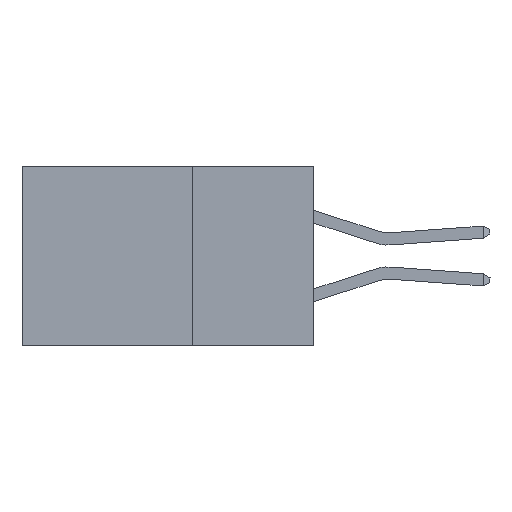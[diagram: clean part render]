
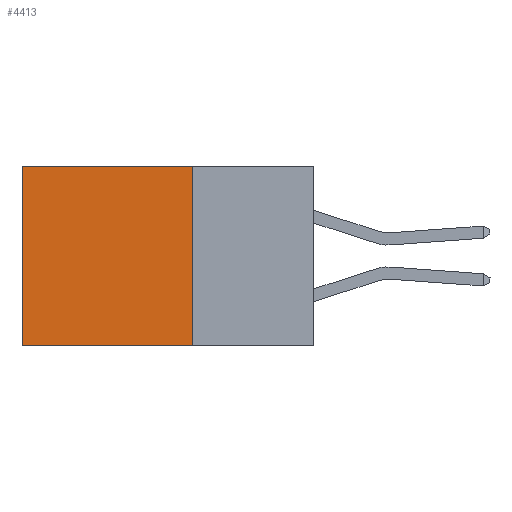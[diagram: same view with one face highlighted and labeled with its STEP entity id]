
A CAD part, left-side view. The second image highlights one B-rep face of the part: STEP entity #4413.
In plain terms, the highlighted planar face has unit normal (-1, 0, 0).
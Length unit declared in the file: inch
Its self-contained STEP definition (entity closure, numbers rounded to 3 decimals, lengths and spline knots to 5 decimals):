
#1766 = LINE ( 'NONE', #30294, #40866 ) ;
#2473 = VECTOR ( 'NONE', #16940, 39.37008 ) ;
#4413 = ADVANCED_FACE ( 'NONE', ( #20172 ), #21716, .F. ) ;
#6239 = LINE ( 'NONE', #27927, #40745 ) ;
#7944 = VERTEX_POINT ( 'NONE', #8410 ) ;
#8410 = CARTESIAN_POINT ( 'NONE',  ( 0.2875, 0.25, -0.37 ) ) ;
#10194 = LINE ( 'NONE', #26515, #30984 ) ;
#10612 = AXIS2_PLACEMENT_3D ( 'NONE', #28231, #31484, #38134 ) ;
#11607 = LINE ( 'NONE', #26440, #2473 ) ;
#13371 = ORIENTED_EDGE ( 'NONE', *, *, #39893, .T. ) ;
#14934 = VERTEX_POINT ( 'NONE', #36385 ) ;
#16940 = DIRECTION ( 'NONE',  ( 0., 1., 0. ) ) ;
#17429 = EDGE_CURVE ( 'NONE', #19860, #26643, #11607, .T. ) ;
#19133 = CARTESIAN_POINT ( 'NONE',  ( 0.2875, 0.25, 0. ) ) ;
#19860 = VERTEX_POINT ( 'NONE', #19133 ) ;
#20172 = FACE_OUTER_BOUND ( 'NONE', #28257, .T. ) ;
#21716 = PLANE ( 'NONE',  #10612 ) ;
#23634 = EDGE_CURVE ( 'NONE', #19860, #7944, #10194, .T. ) ;
#26440 = CARTESIAN_POINT ( 'NONE',  ( 0.2875, 0.25, 0. ) ) ;
#26515 = CARTESIAN_POINT ( 'NONE',  ( 0.2875, 0.25, 0. ) ) ;
#26643 = VERTEX_POINT ( 'NONE', #27523 ) ;
#26904 = DIRECTION ( 'NONE',  ( 0., 0., -1. ) ) ;
#27523 = CARTESIAN_POINT ( 'NONE',  ( 0.2875, 0.6, 0. ) ) ;
#27927 = CARTESIAN_POINT ( 'NONE',  ( 0.2875, 0.25, -0.37 ) ) ;
#28231 = CARTESIAN_POINT ( 'NONE',  ( 0.2875, 0.25, 0. ) ) ;
#28257 = EDGE_LOOP ( 'NONE', ( #13371, #40762, #30875, #31492 ) ) ;
#30294 = CARTESIAN_POINT ( 'NONE',  ( 0.2875, 0.6, 0. ) ) ;
#30307 = DIRECTION ( 'NONE',  ( 0., 0., -1. ) ) ;
#30875 = ORIENTED_EDGE ( 'NONE', *, *, #23634, .F. ) ;
#30984 = VECTOR ( 'NONE', #30307, 39.37008 ) ;
#31484 = DIRECTION ( 'NONE',  ( 1., 0., 0. ) ) ;
#31492 = ORIENTED_EDGE ( 'NONE', *, *, #17429, .T. ) ;
#36369 = EDGE_CURVE ( 'NONE', #7944, #14934, #6239, .T. ) ;
#36385 = CARTESIAN_POINT ( 'NONE',  ( 0.2875, 0.6, -0.37 ) ) ;
#37660 = DIRECTION ( 'NONE',  ( 0., 1., 0. ) ) ;
#38134 = DIRECTION ( 'NONE',  ( 0., 0., -1. ) ) ;
#39893 = EDGE_CURVE ( 'NONE', #26643, #14934, #1766, .T. ) ;
#40745 = VECTOR ( 'NONE', #37660, 39.37008 ) ;
#40762 = ORIENTED_EDGE ( 'NONE', *, *, #36369, .F. ) ;
#40866 = VECTOR ( 'NONE', #26904, 39.37008 ) ;
